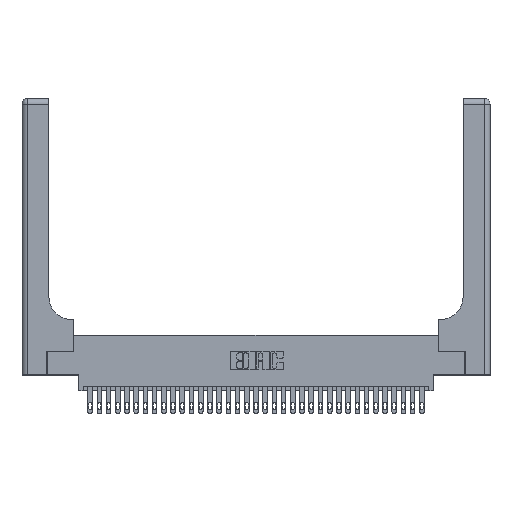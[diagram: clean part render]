
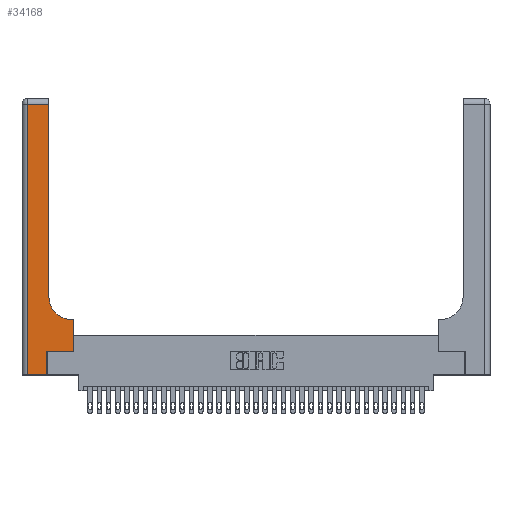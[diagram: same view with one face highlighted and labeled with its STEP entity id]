
A CAD part, top view. The second image highlights one B-rep face of the part: STEP entity #34168.
In plain terms, the highlighted planar face has unit normal (0, 0, 1).
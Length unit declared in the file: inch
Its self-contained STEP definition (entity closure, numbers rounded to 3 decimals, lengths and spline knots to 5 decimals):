
#78 = LINE ( 'NONE', #29648, #10216 ) ;
#240 = EDGE_CURVE ( 'NONE', #19621, #28083, #78, .T. ) ;
#368 = VECTOR ( 'NONE', #3460, 39.37008 ) ;
#506 = ORIENTED_EDGE ( 'NONE', *, *, #15099, .T. ) ;
#1035 = CARTESIAN_POINT ( 'NONE',  ( 0., 3., 0.37 ) ) ;
#2715 = LINE ( 'NONE', #20383, #30605 ) ;
#2838 = CARTESIAN_POINT ( 'NONE',  ( 0.2915, 0.6, 0.37 ) ) ;
#2863 = EDGE_CURVE ( 'NONE', #5167, #5720, #4842, .T. ) ;
#3075 = CARTESIAN_POINT ( 'NONE',  ( 0.06, 3., 0.37 ) ) ;
#3460 = DIRECTION ( 'NONE',  ( 0., 1., 0. ) ) ;
#3582 = VERTEX_POINT ( 'NONE', #6259 ) ;
#4110 = LINE ( 'NONE', #3075, #9590 ) ;
#4842 = LINE ( 'NONE', #34671, #5646 ) ;
#4851 = LINE ( 'NONE', #2838, #32721 ) ;
#5167 = VERTEX_POINT ( 'NONE', #33880 ) ;
#5565 = EDGE_CURVE ( 'NONE', #33205, #19855, #10096, .T. ) ;
#5646 = VECTOR ( 'NONE', #18592, 39.37008 ) ;
#5720 = VERTEX_POINT ( 'NONE', #9355 ) ;
#6259 = CARTESIAN_POINT ( 'NONE',  ( 0.2915, 0.85, 0.37 ) ) ;
#7318 = CARTESIAN_POINT ( 'NONE',  ( 0.5585, 0.6, 0.37 ) ) ;
#7701 = EDGE_CURVE ( 'NONE', #5720, #33205, #4110, .T. ) ;
#8772 = CIRCLE ( 'NONE', #12718, 0.25 ) ;
#8964 = ORIENTED_EDGE ( 'NONE', *, *, #7701, .T. ) ;
#9355 = CARTESIAN_POINT ( 'NONE',  ( 0.06, 2.94, 0.37 ) ) ;
#9555 = CARTESIAN_POINT ( 'NONE',  ( 0.06, 0., 0.37 ) ) ;
#9590 = VECTOR ( 'NONE', #27774, 39.37008 ) ;
#10096 = LINE ( 'NONE', #25105, #19809 ) ;
#10216 = VECTOR ( 'NONE', #28330, 39.37008 ) ;
#10247 = EDGE_CURVE ( 'NONE', #19855, #22346, #23705, .T. ) ;
#11821 = CARTESIAN_POINT ( 'NONE',  ( 0.269, 0.25, 0.37 ) ) ;
#12718 = AXIS2_PLACEMENT_3D ( 'NONE', #34403, #18221, #25435 ) ;
#13127 = EDGE_CURVE ( 'NONE', #28083, #15858, #4851, .T. ) ;
#14136 = DIRECTION ( 'NONE',  ( 0., 0., -1. ) ) ;
#14618 = ORIENTED_EDGE ( 'NONE', *, *, #2863, .T. ) ;
#15071 = DIRECTION ( 'NONE',  ( 0., 1., 0. ) ) ;
#15099 = EDGE_CURVE ( 'NONE', #22346, #19621, #20005, .T. ) ;
#15858 = VERTEX_POINT ( 'NONE', #17956 ) ;
#17956 = CARTESIAN_POINT ( 'NONE',  ( 0.5415, 0.6, 0.37 ) ) ;
#18221 = DIRECTION ( 'NONE',  ( 0., 0., -1. ) ) ;
#18250 = ORIENTED_EDGE ( 'NONE', *, *, #13127, .T. ) ;
#18592 = DIRECTION ( 'NONE',  ( -1., 0., 0. ) ) ;
#18709 = ORIENTED_EDGE ( 'NONE', *, *, #25654, .T. ) ;
#19621 = VERTEX_POINT ( 'NONE', #30300 ) ;
#19660 = DIRECTION ( 'NONE',  ( 1., 0., 0. ) ) ;
#19809 = VECTOR ( 'NONE', #19660, 39.37008 ) ;
#19855 = VERTEX_POINT ( 'NONE', #34060 ) ;
#20005 = LINE ( 'NONE', #24576, #24668 ) ;
#20383 = CARTESIAN_POINT ( 'NONE',  ( 0.2915, 3., 0.37 ) ) ;
#20664 = FACE_OUTER_BOUND ( 'NONE', #22099, .T. ) ;
#21881 = ORIENTED_EDGE ( 'NONE', *, *, #22274, .T. ) ;
#22099 = EDGE_LOOP ( 'NONE', ( #21881, #14618, #8964, #28667, #26984, #506, #24057, #18250, #18709 ) ) ;
#22274 = EDGE_CURVE ( 'NONE', #3582, #5167, #2715, .T. ) ;
#22317 = DIRECTION ( 'NONE',  ( -1., 0., 0. ) ) ;
#22346 = VERTEX_POINT ( 'NONE', #11821 ) ;
#23705 = LINE ( 'NONE', #32869, #368 ) ;
#24057 = ORIENTED_EDGE ( 'NONE', *, *, #240, .T. ) ;
#24576 = CARTESIAN_POINT ( 'NONE',  ( 0.269, 0.25, 0.37 ) ) ;
#24668 = VECTOR ( 'NONE', #28917, 39.37008 ) ;
#25105 = CARTESIAN_POINT ( 'NONE',  ( 0., 0., 0.37 ) ) ;
#25435 = DIRECTION ( 'NONE',  ( 1., 0., 0. ) ) ;
#25654 = EDGE_CURVE ( 'NONE', #15858, #3582, #8772, .T. ) ;
#26984 = ORIENTED_EDGE ( 'NONE', *, *, #10247, .T. ) ;
#27774 = DIRECTION ( 'NONE',  ( 0., -1., 0. ) ) ;
#28083 = VERTEX_POINT ( 'NONE', #7318 ) ;
#28114 = PLANE ( 'NONE',  #32348 ) ;
#28330 = DIRECTION ( 'NONE',  ( 0., 1., 0. ) ) ;
#28667 = ORIENTED_EDGE ( 'NONE', *, *, #5565, .T. ) ;
#28917 = DIRECTION ( 'NONE',  ( 1., 0., 0. ) ) ;
#29648 = CARTESIAN_POINT ( 'NONE',  ( 0.5585, 0.25, 0.37 ) ) ;
#30300 = CARTESIAN_POINT ( 'NONE',  ( 0.5585, 0.25, 0.37 ) ) ;
#30605 = VECTOR ( 'NONE', #15071, 39.37008 ) ;
#32348 = AXIS2_PLACEMENT_3D ( 'NONE', #1035, #14136, #22317 ) ;
#32721 = VECTOR ( 'NONE', #33524, 39.37008 ) ;
#32869 = CARTESIAN_POINT ( 'NONE',  ( 0.269, 0., 0.37 ) ) ;
#33205 = VERTEX_POINT ( 'NONE', #9555 ) ;
#33524 = DIRECTION ( 'NONE',  ( -1., 0., 0. ) ) ;
#33880 = CARTESIAN_POINT ( 'NONE',  ( 0.2915, 2.94, 0.37 ) ) ;
#34060 = CARTESIAN_POINT ( 'NONE',  ( 0.269, 0., 0.37 ) ) ;
#34168 = ADVANCED_FACE ( 'NONE', ( #20664 ), #28114, .F. ) ;
#34403 = CARTESIAN_POINT ( 'NONE',  ( 0.5415, 0.85, 0.37 ) ) ;
#34671 = CARTESIAN_POINT ( 'NONE',  ( 0., 2.94, 0.37 ) ) ;
